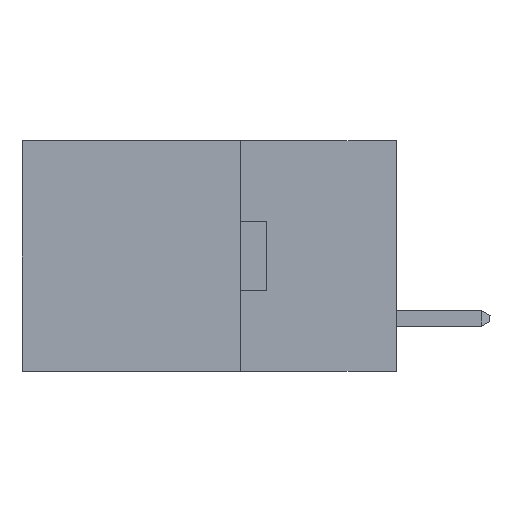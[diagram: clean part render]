
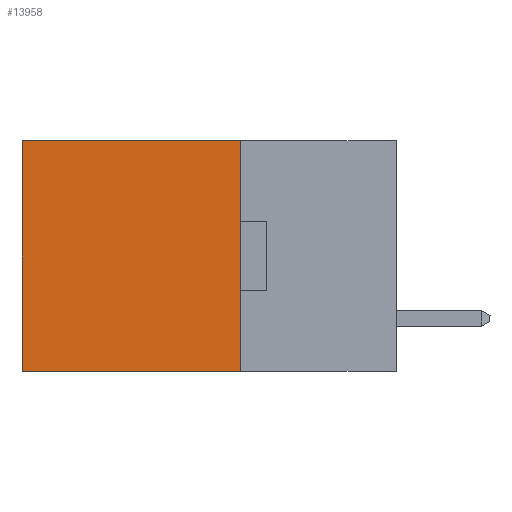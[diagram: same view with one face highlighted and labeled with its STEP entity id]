
A CAD part, left-side view. The second image highlights one B-rep face of the part: STEP entity #13958.
In plain terms, the highlighted planar face has unit normal (-1, 0, 0).
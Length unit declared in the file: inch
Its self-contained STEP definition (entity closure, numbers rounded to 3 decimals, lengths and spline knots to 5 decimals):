
#813 = LINE ( 'NONE', #16714, #11625 ) ;
#875 = DIRECTION ( 'NONE',  ( 0., 0., -1. ) ) ;
#1361 = CARTESIAN_POINT ( 'NONE',  ( 0.2615, 0.25, 0. ) ) ;
#1905 = DIRECTION ( 'NONE',  ( 1., 0., 0. ) ) ;
#2096 = DIRECTION ( 'NONE',  ( 0., 0., -1. ) ) ;
#2457 = VECTOR ( 'NONE', #9965, 39.37008 ) ;
#4689 = ORIENTED_EDGE ( 'NONE', *, *, #21349, .T. ) ;
#5343 = AXIS2_PLACEMENT_3D ( 'NONE', #27177, #1905, #16960 ) ;
#6819 = VECTOR ( 'NONE', #875, 39.37008 ) ;
#8388 = VERTEX_POINT ( 'NONE', #10248 ) ;
#9373 = EDGE_LOOP ( 'NONE', ( #4689, #14521, #23844, #14602 ) ) ;
#9965 = DIRECTION ( 'NONE',  ( 0., 1., 0. ) ) ;
#10248 = CARTESIAN_POINT ( 'NONE',  ( 0.2615, 0.25, -0.37 ) ) ;
#10520 = PLANE ( 'NONE',  #5343 ) ;
#11221 = VERTEX_POINT ( 'NONE', #11631 ) ;
#11625 = VECTOR ( 'NONE', #25004, 39.37008 ) ;
#11631 = CARTESIAN_POINT ( 'NONE',  ( 0.2615, 0.6, -0.37 ) ) ;
#11658 = CARTESIAN_POINT ( 'NONE',  ( 0.2615, 0.25, 0. ) ) ;
#12827 = CARTESIAN_POINT ( 'NONE',  ( 0.2615, 0.6, -0.37 ) ) ;
#13775 = CARTESIAN_POINT ( 'NONE',  ( 0.2615, 0.25, -0.37 ) ) ;
#13958 = ADVANCED_FACE ( 'NONE', ( #17525 ), #10520, .F. ) ;
#14521 = ORIENTED_EDGE ( 'NONE', *, *, #23760, .F. ) ;
#14602 = ORIENTED_EDGE ( 'NONE', *, *, #18970, .T. ) ;
#15967 = VERTEX_POINT ( 'NONE', #19147 ) ;
#16714 = CARTESIAN_POINT ( 'NONE',  ( 0.2615, 0.25, -0.37 ) ) ;
#16960 = DIRECTION ( 'NONE',  ( 0., 0., -1. ) ) ;
#17525 = FACE_OUTER_BOUND ( 'NONE', #9373, .T. ) ;
#18880 = LINE ( 'NONE', #1361, #2457 ) ;
#18970 = EDGE_CURVE ( 'NONE', #20453, #15967, #18880, .T. ) ;
#19147 = CARTESIAN_POINT ( 'NONE',  ( 0.2615, 0.6, 0. ) ) ;
#20453 = VERTEX_POINT ( 'NONE', #11658 ) ;
#21349 = EDGE_CURVE ( 'NONE', #15967, #11221, #23590, .T. ) ;
#22306 = VECTOR ( 'NONE', #2096, 39.37008 ) ;
#23590 = LINE ( 'NONE', #12827, #22306 ) ;
#23760 = EDGE_CURVE ( 'NONE', #8388, #11221, #813, .T. ) ;
#23844 = ORIENTED_EDGE ( 'NONE', *, *, #26015, .F. ) ;
#24313 = LINE ( 'NONE', #13775, #6819 ) ;
#25004 = DIRECTION ( 'NONE',  ( 0., 1., 0. ) ) ;
#26015 = EDGE_CURVE ( 'NONE', #20453, #8388, #24313, .T. ) ;
#27177 = CARTESIAN_POINT ( 'NONE',  ( 0.2615, 0.25, -0.37 ) ) ;
